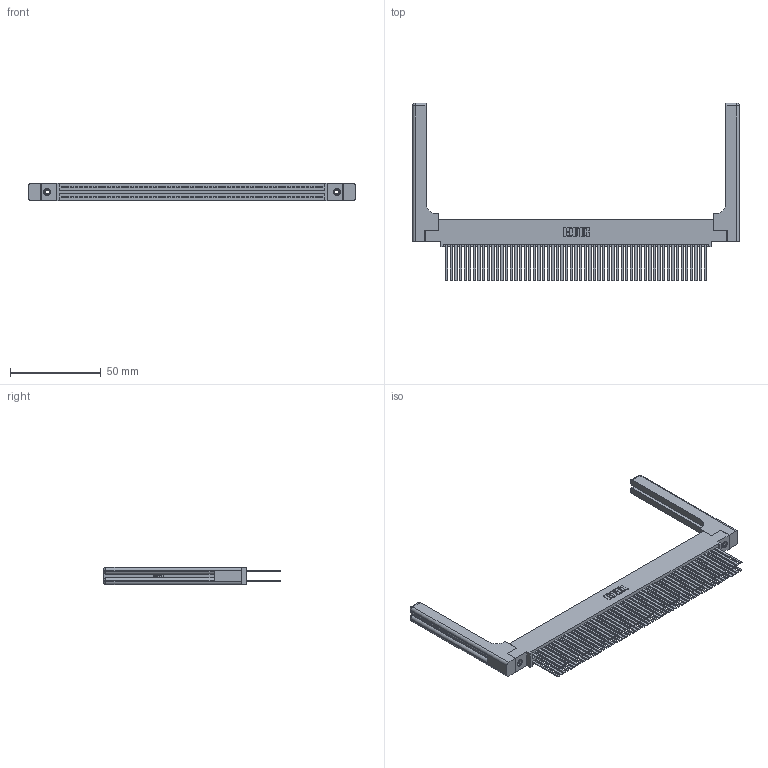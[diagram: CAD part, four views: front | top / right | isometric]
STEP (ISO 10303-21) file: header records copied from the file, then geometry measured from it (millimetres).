
FILE_DESCRIPTION (( 'STEP AP203' ), '1' );
FILE_NAME ('395-114-544-558.STEP', '2019-10-27T18:36:34', ( '' ), ( '' ), 'SwSTEP 2.0', 'SolidWorks 2016', '' );
FILE_SCHEMA (( 'CONFIG_CONTROL_DESIGN' ));
Length unit declared in the file: inch
Products named in the file (5): 395-114-544-558; 345 Part_0.110 Offset - 0.156 Dia-TH; 345-292-001_345-293-144; 345-250-001_345-250-001-102; 345-220-058_345-220-058
Assembly tree (119 placements, depth 2):
  395-114-544-558
    345 Part_0.110 Offset - 0.156 Dia-TH
    345-292-001_345-293-144  x114
    345-250-001_345-250-001-102  x2
    345-220-058_345-220-058  x2
Bounding box: 179.81 x 97.71 x 9.4 mm (x, y, z)
Volume: 27605.6 mm3; surface area: 38404.2 mm2
Topology: 119 solids, 119 shells, 5402 faces, 15953 edges, 10462 vertices
Faces by surface type: plane 3538, cylinder 1804, bspline 36, cone 12, sphere 8, torus 4
Entity records: 47834 total; most frequent: CARTESIAN_POINT 8997, ORIENTED_EDGE 7728, DIRECTION 6844, EDGE_CURVE 3864, LINE 3416, VECTOR 3416, VERTEX_POINT 2566, AXIS2_PLACEMENT_3D 1714
